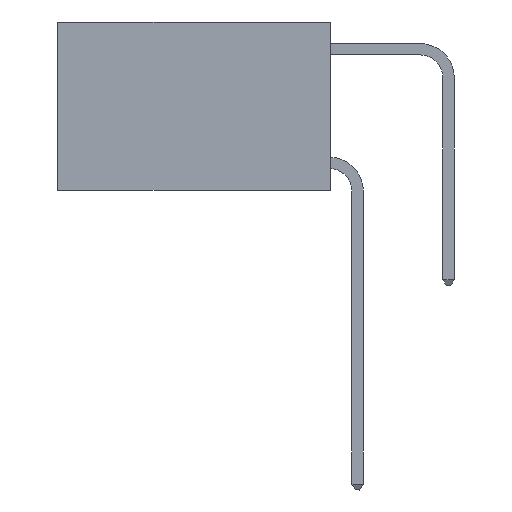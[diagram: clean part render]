
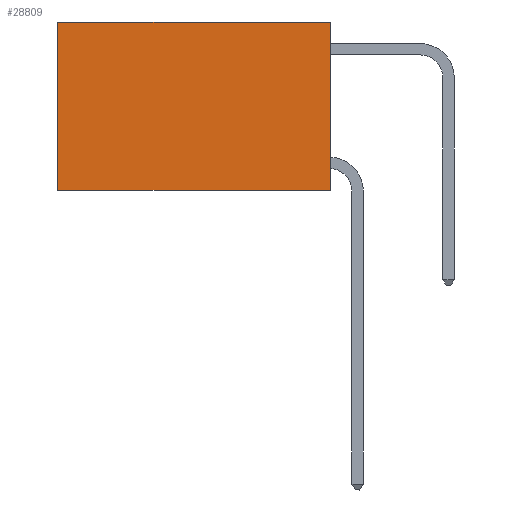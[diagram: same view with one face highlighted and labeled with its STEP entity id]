
A CAD part, left-side view. The second image highlights one B-rep face of the part: STEP entity #28809.
In plain terms, the highlighted planar face has unit normal (-1, 0, 0).
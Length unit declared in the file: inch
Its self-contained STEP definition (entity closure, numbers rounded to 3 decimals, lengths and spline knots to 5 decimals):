
#517 = VERTEX_POINT ( 'NONE', #26433 ) ;
#1012 = EDGE_CURVE ( 'NONE', #23693, #517, #9288, .T. ) ;
#1770 = ORIENTED_EDGE ( 'NONE', *, *, #22309, .T. ) ;
#2205 = CARTESIAN_POINT ( 'NONE',  ( 0.2625, 0., -0.37 ) ) ;
#2538 = PLANE ( 'NONE',  #10272 ) ;
#3074 = EDGE_CURVE ( 'NONE', #23237, #517, #4622, .T. ) ;
#3155 = CARTESIAN_POINT ( 'NONE',  ( 0.2625, 0., -0.37 ) ) ;
#4398 = VECTOR ( 'NONE', #12994, 39.37008 ) ;
#4622 = LINE ( 'NONE', #3155, #16681 ) ;
#4767 = ORIENTED_EDGE ( 'NONE', *, *, #1012, .T. ) ;
#7156 = CARTESIAN_POINT ( 'NONE',  ( 0.2625, 0., 0. ) ) ;
#7397 = DIRECTION ( 'NONE',  ( 0., 0., -1. ) ) ;
#8248 = FACE_OUTER_BOUND ( 'NONE', #25131, .T. ) ;
#9288 = LINE ( 'NONE', #11564, #21352 ) ;
#9559 = DIRECTION ( 'NONE',  ( 0., 0., -1. ) ) ;
#9614 = CARTESIAN_POINT ( 'NONE',  ( 0.2625, 0.6, 0. ) ) ;
#10272 = AXIS2_PLACEMENT_3D ( 'NONE', #19435, #21813, #7397 ) ;
#11564 = CARTESIAN_POINT ( 'NONE',  ( 0.2625, 0.6, 0. ) ) ;
#12418 = ORIENTED_EDGE ( 'NONE', *, *, #3074, .F. ) ;
#12994 = DIRECTION ( 'NONE',  ( 0., 1., 0. ) ) ;
#13954 = DIRECTION ( 'NONE',  ( 0., 0., -1. ) ) ;
#15383 = ORIENTED_EDGE ( 'NONE', *, *, #29390, .F. ) ;
#15724 = VECTOR ( 'NONE', #9559, 39.37008 ) ;
#16681 = VECTOR ( 'NONE', #20054, 39.37008 ) ;
#19435 = CARTESIAN_POINT ( 'NONE',  ( 0.2625, 0., 0. ) ) ;
#20054 = DIRECTION ( 'NONE',  ( 0., 1., 0. ) ) ;
#21352 = VECTOR ( 'NONE', #13954, 39.37008 ) ;
#21813 = DIRECTION ( 'NONE',  ( 1., 0., 0. ) ) ;
#22309 = EDGE_CURVE ( 'NONE', #27626, #23693, #23594, .T. ) ;
#23237 = VERTEX_POINT ( 'NONE', #2205 ) ;
#23594 = LINE ( 'NONE', #27337, #4398 ) ;
#23693 = VERTEX_POINT ( 'NONE', #9614 ) ;
#24878 = CARTESIAN_POINT ( 'NONE',  ( 0.2625, 0., 0. ) ) ;
#25131 = EDGE_LOOP ( 'NONE', ( #4767, #12418, #15383, #1770 ) ) ;
#26433 = CARTESIAN_POINT ( 'NONE',  ( 0.2625, 0.6, -0.37 ) ) ;
#27337 = CARTESIAN_POINT ( 'NONE',  ( 0.2625, 0., 0. ) ) ;
#27626 = VERTEX_POINT ( 'NONE', #24878 ) ;
#28418 = LINE ( 'NONE', #7156, #15724 ) ;
#28809 = ADVANCED_FACE ( 'NONE', ( #8248 ), #2538, .F. ) ;
#29390 = EDGE_CURVE ( 'NONE', #27626, #23237, #28418, .T. ) ;
